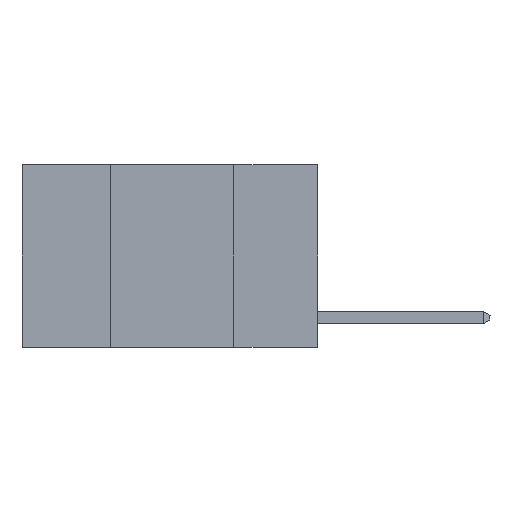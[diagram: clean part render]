
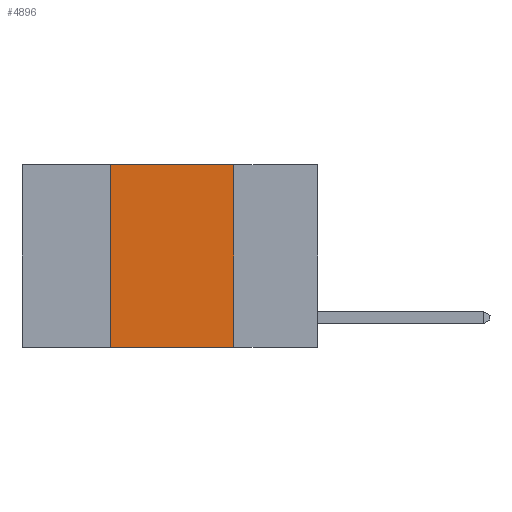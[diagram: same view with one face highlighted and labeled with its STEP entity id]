
A CAD part, left-side view. The second image highlights one B-rep face of the part: STEP entity #4896.
In plain terms, the highlighted planar face has unit normal (-1, 0, 0).
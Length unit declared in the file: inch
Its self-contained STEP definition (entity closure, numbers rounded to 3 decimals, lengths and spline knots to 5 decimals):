
#318 = ORIENTED_EDGE ( 'NONE', *, *, #5809, .F. ) ;
#409 = LINE ( 'NONE', #8761, #3876 ) ;
#1405 = VECTOR ( 'NONE', #10954, 39.37008 ) ;
#1454 = CARTESIAN_POINT ( 'NONE',  ( 0., 0.17, 0. ) ) ;
#2829 = VECTOR ( 'NONE', #12542, 39.37008 ) ;
#3006 = ORIENTED_EDGE ( 'NONE', *, *, #10042, .F. ) ;
#3081 = ORIENTED_EDGE ( 'NONE', *, *, #9312, .T. ) ;
#3579 = PLANE ( 'NONE',  #6050 ) ;
#3876 = VECTOR ( 'NONE', #7638, 39.37008 ) ;
#4896 = ADVANCED_FACE ( 'NONE', ( #6579 ), #3579, .F. ) ;
#5809 = EDGE_CURVE ( 'NONE', #9805, #5892, #409, .T. ) ;
#5891 = DIRECTION ( 'NONE',  ( 1., 0., 0. ) ) ;
#5892 = VERTEX_POINT ( 'NONE', #8904 ) ;
#5988 = CARTESIAN_POINT ( 'NONE',  ( 0., 0.42, 0. ) ) ;
#6050 = AXIS2_PLACEMENT_3D ( 'NONE', #11358, #5891, #13540 ) ;
#6579 = FACE_OUTER_BOUND ( 'NONE', #11051, .T. ) ;
#7638 = DIRECTION ( 'NONE',  ( 0., -1., 0. ) ) ;
#8635 = CARTESIAN_POINT ( 'NONE',  ( 0., 0.42, 0. ) ) ;
#8761 = CARTESIAN_POINT ( 'NONE',  ( 0., 0.6, 0. ) ) ;
#8847 = LINE ( 'NONE', #5988, #2829 ) ;
#8904 = CARTESIAN_POINT ( 'NONE',  ( 0., 0.17, 0. ) ) ;
#9312 = EDGE_CURVE ( 'NONE', #11846, #10259, #12953, .T. ) ;
#9340 = DIRECTION ( 'NONE',  ( 0., 0., -1. ) ) ;
#9637 = CARTESIAN_POINT ( 'NONE',  ( 0., 0.17, -0.37 ) ) ;
#9805 = VERTEX_POINT ( 'NONE', #8635 ) ;
#10042 = EDGE_CURVE ( 'NONE', #11846, #9805, #8847, .T. ) ;
#10259 = VERTEX_POINT ( 'NONE', #9637 ) ;
#10782 = EDGE_CURVE ( 'NONE', #5892, #10259, #13758, .T. ) ;
#10885 = VECTOR ( 'NONE', #9340, 39.37008 ) ;
#10954 = DIRECTION ( 'NONE',  ( 0., -1., 0. ) ) ;
#11051 = EDGE_LOOP ( 'NONE', ( #13788, #318, #3006, #3081 ) ) ;
#11080 = CARTESIAN_POINT ( 'NONE',  ( 0., 0.42, -0.37 ) ) ;
#11358 = CARTESIAN_POINT ( 'NONE',  ( 0., 0.6, 0. ) ) ;
#11846 = VERTEX_POINT ( 'NONE', #11080 ) ;
#12542 = DIRECTION ( 'NONE',  ( 0., 0., 1. ) ) ;
#12953 = LINE ( 'NONE', #14237, #1405 ) ;
#13540 = DIRECTION ( 'NONE',  ( 0., 0., -1. ) ) ;
#13758 = LINE ( 'NONE', #1454, #10885 ) ;
#13788 = ORIENTED_EDGE ( 'NONE', *, *, #10782, .F. ) ;
#14237 = CARTESIAN_POINT ( 'NONE',  ( 0., 0.6, -0.37 ) ) ;
